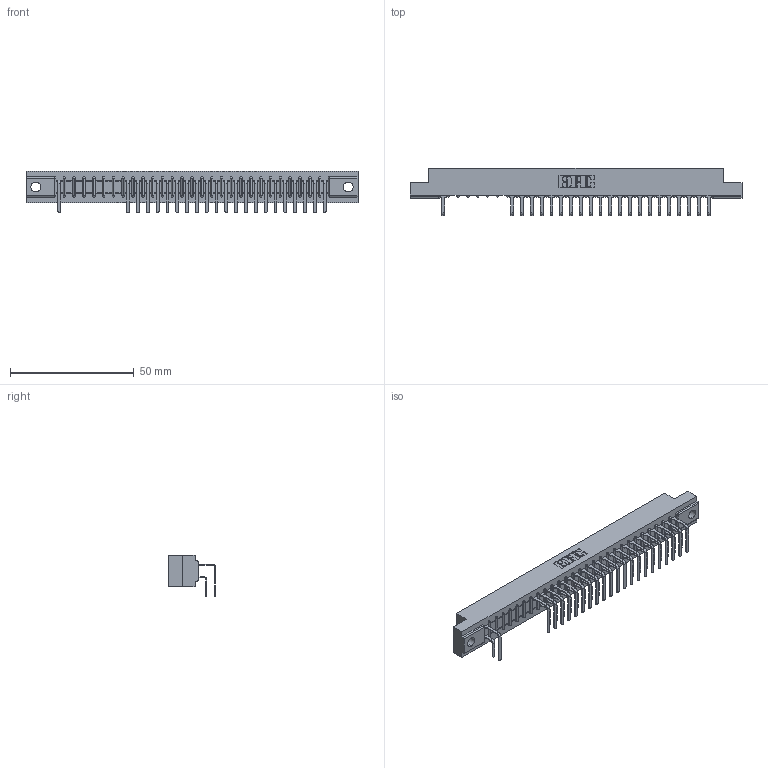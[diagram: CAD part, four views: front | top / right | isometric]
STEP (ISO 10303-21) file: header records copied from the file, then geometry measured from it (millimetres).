
FILE_DESCRIPTION (( 'STEP AP203' ), '1' );
FILE_NAME ('307-056-558-204.STEP', '2018-08-06T07:05:05', ( '' ), ( '' ), 'SwSTEP 2.0', 'SolidWorks 2016', '' );
FILE_SCHEMA (( 'CONFIG_CONTROL_DESIGN' ));
Length unit declared in the file: inch
Products named in the file (4): 307-056-558-204; 307 Part_.156 Dia Mounting Holes; 307-290-001_558 559 - 1 (Single); 307-290-001_558 - 2 (Single)
Assembly tree (44 placements, depth 2):
  307-056-558-204
    307 Part_.156 Dia Mounting Holes
    307-290-001_558 559 - 1 (Single)  x21
    307-290-001_558 - 2 (Single)  x22
Bounding box: 133.96 x 18.96 x 16.8 mm (x, y, z)
Volume: 14063.8 mm3; surface area: 16774.9 mm2
Topology: 44 solids, 44 shells, 2441 faces, 6881 edges, 4450 vertices
Faces by surface type: plane 1581, cylinder 802, sphere 58
Entity records: 28075 total; most frequent: CARTESIAN_POINT 4659, ORIENTED_EDGE 4626, DIRECTION 4547, EDGE_CURVE 2313, VECTOR 1775, LINE 1775, VERTEX_POINT 1498, AXIS2_PLACEMENT_3D 1386
